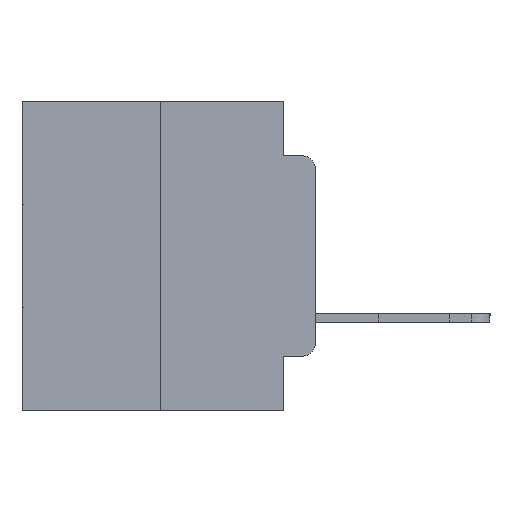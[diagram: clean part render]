
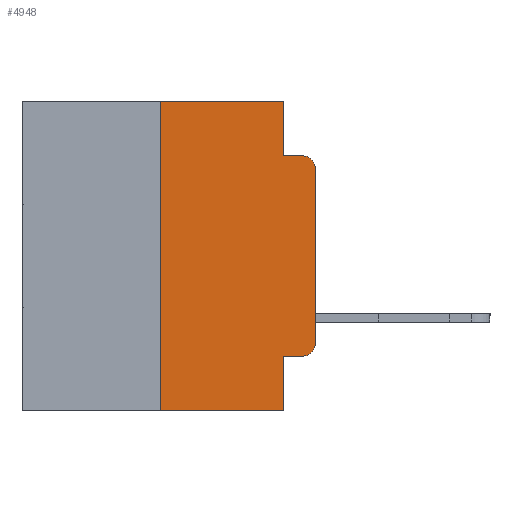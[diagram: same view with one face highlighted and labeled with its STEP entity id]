
A CAD part, left-side view. The second image highlights one B-rep face of the part: STEP entity #4948.
In plain terms, the highlighted planar face has unit normal (-1, 0, 0).
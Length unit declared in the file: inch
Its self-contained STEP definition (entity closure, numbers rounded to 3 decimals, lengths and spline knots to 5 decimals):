
#747 = ORIENTED_EDGE ( 'NONE', *, *, #2882, .F. ) ;
#788 = DIRECTION ( 'NONE',  ( 1., 0., 0. ) ) ;
#834 = LINE ( 'NONE', #1132, #6406 ) ;
#971 = CARTESIAN_POINT ( 'NONE',  ( 0., 0.051, -0.4115 ) ) ;
#1132 = CARTESIAN_POINT ( 'NONE',  ( 0., 0., 0. ) ) ;
#2211 = CIRCLE ( 'NONE', #21753, 0.02 ) ;
#2381 = CARTESIAN_POINT ( 'NONE',  ( 0., 0.051, 0. ) ) ;
#2427 = VERTEX_POINT ( 'NONE', #4021 ) ;
#2745 = DIRECTION ( 'NONE',  ( -1., 0., 0. ) ) ;
#2853 = EDGE_CURVE ( 'NONE', #8176, #2427, #20717, .T. ) ;
#2882 = EDGE_CURVE ( 'NONE', #16085, #2427, #14181, .T. ) ;
#3214 = EDGE_CURVE ( 'NONE', #6967, #21006, #22469, .T. ) ;
#3732 = VECTOR ( 'NONE', #22234, 39.37008 ) ;
#4021 = CARTESIAN_POINT ( 'NONE',  ( 0., 0.051, -0.5 ) ) ;
#4530 = VERTEX_POINT ( 'NONE', #25356 ) ;
#4948 = ADVANCED_FACE ( 'NONE', ( #5020 ), #15650, .F. ) ;
#4992 = ORIENTED_EDGE ( 'NONE', *, *, #21748, .F. ) ;
#5020 = FACE_OUTER_BOUND ( 'NONE', #16639, .T. ) ;
#5655 = CARTESIAN_POINT ( 'NONE',  ( 0., 0.02, -0.1085 ) ) ;
#5852 = LINE ( 'NONE', #25793, #25919 ) ;
#6406 = VECTOR ( 'NONE', #15648, 39.37008 ) ;
#6640 = ORIENTED_EDGE ( 'NONE', *, *, #21185, .T. ) ;
#6967 = VERTEX_POINT ( 'NONE', #2381 ) ;
#7201 = EDGE_CURVE ( 'NONE', #16085, #12620, #7243, .T. ) ;
#7243 = LINE ( 'NONE', #19445, #18105 ) ;
#7272 = VERTEX_POINT ( 'NONE', #23564 ) ;
#7327 = DIRECTION ( 'NONE',  ( 0., -1., 0. ) ) ;
#7350 = VECTOR ( 'NONE', #17368, 39.37008 ) ;
#7764 = DIRECTION ( 'NONE',  ( 0., 0., -1. ) ) ;
#8176 = VERTEX_POINT ( 'NONE', #16871 ) ;
#8447 = CARTESIAN_POINT ( 'NONE',  ( 0., 0., -0.3915 ) ) ;
#8564 = EDGE_CURVE ( 'NONE', #21006, #4530, #5852, .T. ) ;
#8734 = VERTEX_POINT ( 'NONE', #8447 ) ;
#8886 = EDGE_CURVE ( 'NONE', #12620, #8734, #2211, .T. ) ;
#9038 = AXIS2_PLACEMENT_3D ( 'NONE', #5655, #19935, #7764 ) ;
#10163 = LINE ( 'NONE', #17651, #14956 ) ;
#10610 = DIRECTION ( 'NONE',  ( 0., 0., -1. ) ) ;
#10727 = CARTESIAN_POINT ( 'NONE',  ( 0., 0.473, -0.5 ) ) ;
#11879 = ORIENTED_EDGE ( 'NONE', *, *, #8886, .T. ) ;
#12019 = DIRECTION ( 'NONE',  ( 0., -1., 0. ) ) ;
#12620 = VERTEX_POINT ( 'NONE', #13483 ) ;
#12848 = ORIENTED_EDGE ( 'NONE', *, *, #8564, .F. ) ;
#13345 = CARTESIAN_POINT ( 'NONE',  ( 0., 0.473, 0. ) ) ;
#13483 = CARTESIAN_POINT ( 'NONE',  ( 0., 0.02, -0.4115 ) ) ;
#14181 = LINE ( 'NONE', #25157, #20096 ) ;
#14425 = AXIS2_PLACEMENT_3D ( 'NONE', #23320, #788, #21153 ) ;
#14577 = EDGE_CURVE ( 'NONE', #21810, #4530, #26227, .T. ) ;
#14956 = VECTOR ( 'NONE', #19663, 39.37008 ) ;
#15190 = CARTESIAN_POINT ( 'NONE',  ( 0., 0.02, -0.3915 ) ) ;
#15648 = DIRECTION ( 'NONE',  ( 0., 0., 1. ) ) ;
#15650 = PLANE ( 'NONE',  #14425 ) ;
#15974 = ORIENTED_EDGE ( 'NONE', *, *, #2853, .T. ) ;
#16085 = VERTEX_POINT ( 'NONE', #971 ) ;
#16639 = EDGE_LOOP ( 'NONE', ( #6640, #23317, #12848, #23929, #4992, #25751, #15974, #747, #21840, #11879 ) ) ;
#16871 = CARTESIAN_POINT ( 'NONE',  ( 0., 0.25, -0.5 ) ) ;
#17186 = DIRECTION ( 'NONE',  ( 0., 0., -1. ) ) ;
#17282 = VECTOR ( 'NONE', #22369, 39.37008 ) ;
#17368 = DIRECTION ( 'NONE',  ( 0., -1., 0. ) ) ;
#17651 = CARTESIAN_POINT ( 'NONE',  ( 0., 0.25, 0. ) ) ;
#18105 = VECTOR ( 'NONE', #7327, 39.37008 ) ;
#18557 = EDGE_CURVE ( 'NONE', #8176, #7272, #10163, .T. ) ;
#19445 = CARTESIAN_POINT ( 'NONE',  ( 0., 0.051, -0.4115 ) ) ;
#19663 = DIRECTION ( 'NONE',  ( 0., 0., 1. ) ) ;
#19935 = DIRECTION ( 'NONE',  ( -1., 0., 0. ) ) ;
#20096 = VECTOR ( 'NONE', #10610, 39.37008 ) ;
#20717 = LINE ( 'NONE', #10727, #3732 ) ;
#21006 = VERTEX_POINT ( 'NONE', #22945 ) ;
#21153 = DIRECTION ( 'NONE',  ( 0., 0., -1. ) ) ;
#21185 = EDGE_CURVE ( 'NONE', #8734, #21810, #834, .T. ) ;
#21748 = EDGE_CURVE ( 'NONE', #7272, #6967, #23380, .T. ) ;
#21753 = AXIS2_PLACEMENT_3D ( 'NONE', #15190, #2745, #17186 ) ;
#21810 = VERTEX_POINT ( 'NONE', #25265 ) ;
#21840 = ORIENTED_EDGE ( 'NONE', *, *, #7201, .T. ) ;
#22234 = DIRECTION ( 'NONE',  ( 0., -1., 0. ) ) ;
#22369 = DIRECTION ( 'NONE',  ( 0., 0., -1. ) ) ;
#22417 = CARTESIAN_POINT ( 'NONE',  ( 0., 0.051, 0. ) ) ;
#22469 = LINE ( 'NONE', #22417, #17282 ) ;
#22945 = CARTESIAN_POINT ( 'NONE',  ( 0., 0.051, -0.0885 ) ) ;
#23317 = ORIENTED_EDGE ( 'NONE', *, *, #14577, .T. ) ;
#23320 = CARTESIAN_POINT ( 'NONE',  ( 0., 0.473, 0. ) ) ;
#23380 = LINE ( 'NONE', #13345, #7350 ) ;
#23564 = CARTESIAN_POINT ( 'NONE',  ( 0., 0.25, 0. ) ) ;
#23929 = ORIENTED_EDGE ( 'NONE', *, *, #3214, .F. ) ;
#25157 = CARTESIAN_POINT ( 'NONE',  ( 0., 0.051, 0. ) ) ;
#25265 = CARTESIAN_POINT ( 'NONE',  ( 0., 0., -0.1085 ) ) ;
#25356 = CARTESIAN_POINT ( 'NONE',  ( 0., 0.02, -0.0885 ) ) ;
#25751 = ORIENTED_EDGE ( 'NONE', *, *, #18557, .F. ) ;
#25793 = CARTESIAN_POINT ( 'NONE',  ( 0., 0.051, -0.0885 ) ) ;
#25919 = VECTOR ( 'NONE', #12019, 39.37008 ) ;
#26227 = CIRCLE ( 'NONE', #9038, 0.02 ) ;
